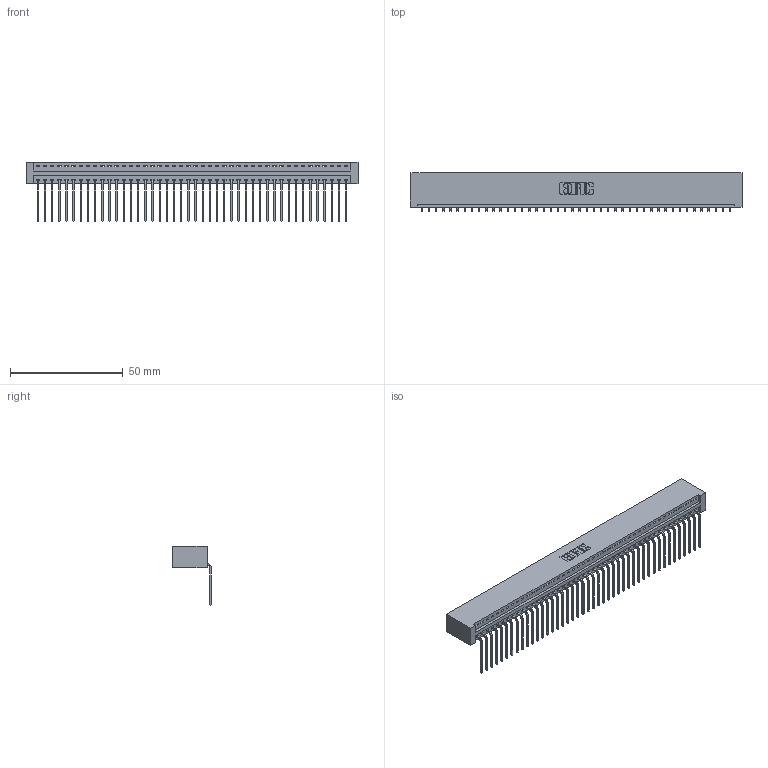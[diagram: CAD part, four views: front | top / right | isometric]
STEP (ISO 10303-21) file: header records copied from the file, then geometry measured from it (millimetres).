
FILE_DESCRIPTION (( 'STEP AP203' ), '1' );
FILE_NAME ('346-044-559-101.STEP', '2018-08-25T02:49:08', ( '' ), ( '' ), 'SwSTEP 2.0', 'SolidWorks 2016', '' );
FILE_SCHEMA (( 'CONFIG_CONTROL_DESIGN' ));
Length unit declared in the file: inch
Products named in the file (3): 346 Part_No Mounting Lugs; 345-292-001_558 559 Tail - 1; 346-044-559-101
Assembly tree (45 placements, depth 2):
  346-044-559-101
    346 Part_No Mounting Lugs
    345-292-001_558 559 Tail - 1  x44
Bounding box: 146.94 x 17.08 x 26.16 mm (x, y, z)
Volume: 14775.1 mm3; surface area: 19438.2 mm2
Topology: 45 solids, 45 shells, 2754 faces, 8313 edges, 5482 vertices
Faces by surface type: plane 1920, cylinder 834
Entity records: 26845 total; most frequent: CARTESIAN_POINT 4608, ORIENTED_EDGE 4586, DIRECTION 4057, EDGE_CURVE 2293, VECTOR 1993, LINE 1993, VERTEX_POINT 1526, AXIS2_PLACEMENT_3D 1032
